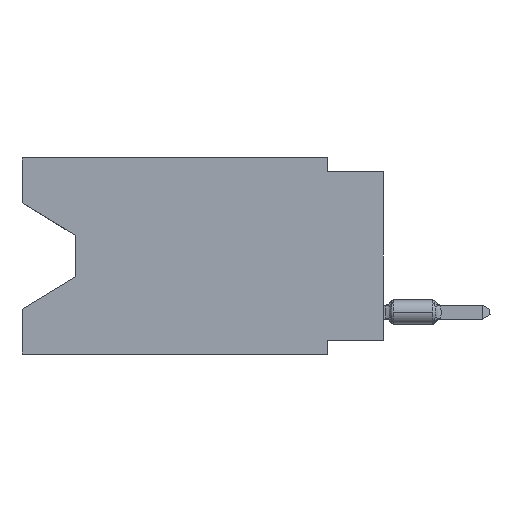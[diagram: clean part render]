
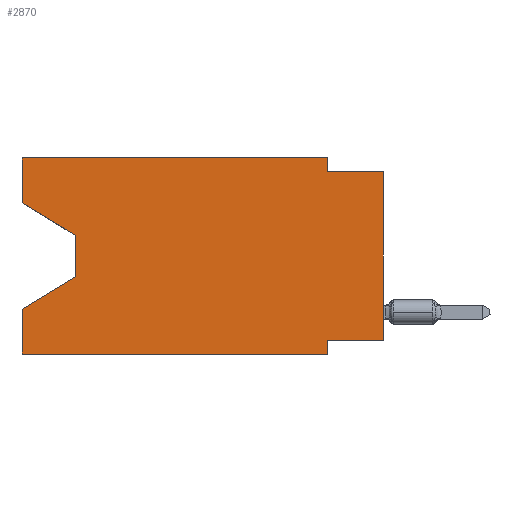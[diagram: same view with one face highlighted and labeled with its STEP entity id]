
A CAD part, left-side view. The second image highlights one B-rep face of the part: STEP entity #2870.
In plain terms, the highlighted planar face has unit normal (-1, 0, 0).
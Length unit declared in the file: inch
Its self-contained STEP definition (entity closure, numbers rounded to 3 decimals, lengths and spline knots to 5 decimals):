
#119 = CARTESIAN_POINT ( 'NONE',  ( 0., 0., -0.025 ) ) ;
#227 = DIRECTION ( 'NONE',  ( 0., 1., 0. ) ) ;
#538 = CARTESIAN_POINT ( 'NONE',  ( 0., 0.645, 0. ) ) ;
#648 = VERTEX_POINT ( 'NONE', #4481 ) ;
#923 = LINE ( 'NONE', #16245, #11190 ) ;
#1853 = VERTEX_POINT ( 'NONE', #9119 ) ;
#1995 = ORIENTED_EDGE ( 'NONE', *, *, #6807, .F. ) ;
#2394 = DIRECTION ( 'NONE',  ( 0., 0., 1. ) ) ;
#2590 = CARTESIAN_POINT ( 'NONE',  ( 0., 0.1, 0. ) ) ;
#2631 = VECTOR ( 'NONE', #4880, 39.37008 ) ;
#2761 = ORIENTED_EDGE ( 'NONE', *, *, #10690, .F. ) ;
#2870 = ADVANCED_FACE ( 'NONE', ( #11526 ), #4623, .F. ) ;
#3121 = LINE ( 'NONE', #119, #16254 ) ;
#3537 = CARTESIAN_POINT ( 'NONE',  ( 0., 0.55, -0.212 ) ) ;
#3776 = LINE ( 'NONE', #10771, #2631 ) ;
#4215 = EDGE_CURVE ( 'NONE', #14684, #5134, #6753, .T. ) ;
#4271 = CARTESIAN_POINT ( 'NONE',  ( 0., 0.645, 0. ) ) ;
#4279 = ORIENTED_EDGE ( 'NONE', *, *, #12678, .F. ) ;
#4481 = CARTESIAN_POINT ( 'NONE',  ( 0., 0.645, -0.08025 ) ) ;
#4498 = DIRECTION ( 'NONE',  ( 0., -1., 0. ) ) ;
#4530 = DIRECTION ( 'NONE',  ( 0., 0., -1. ) ) ;
#4623 = PLANE ( 'NONE',  #16631 ) ;
#4880 = DIRECTION ( 'NONE',  ( 0., 0., 1. ) ) ;
#4951 = CARTESIAN_POINT ( 'NONE',  ( 0., 0.1, -0.35 ) ) ;
#5134 = VERTEX_POINT ( 'NONE', #6136 ) ;
#5175 = CARTESIAN_POINT ( 'NONE',  ( 0., 0.645, -0.35 ) ) ;
#5552 = ORIENTED_EDGE ( 'NONE', *, *, #16722, .T. ) ;
#5636 = VECTOR ( 'NONE', #7919, 39.37008 ) ;
#5731 = EDGE_CURVE ( 'NONE', #13386, #7227, #6645, .T. ) ;
#6094 = CARTESIAN_POINT ( 'NONE',  ( 0., 0.55, -0.138 ) ) ;
#6136 = CARTESIAN_POINT ( 'NONE',  ( 0., 0.645, -0.26975 ) ) ;
#6188 = VERTEX_POINT ( 'NONE', #2590 ) ;
#6567 = CARTESIAN_POINT ( 'NONE',  ( 0., 0.645, 0. ) ) ;
#6645 = LINE ( 'NONE', #16562, #5636 ) ;
#6753 = LINE ( 'NONE', #3537, #9103 ) ;
#6807 = EDGE_CURVE ( 'NONE', #6920, #6188, #11647, .T. ) ;
#6920 = VERTEX_POINT ( 'NONE', #6567 ) ;
#7227 = VERTEX_POINT ( 'NONE', #4951 ) ;
#7360 = DIRECTION ( 'NONE',  ( 1., 0., 0. ) ) ;
#7716 = ORIENTED_EDGE ( 'NONE', *, *, #11211, .T. ) ;
#7802 = ORIENTED_EDGE ( 'NONE', *, *, #4215, .T. ) ;
#7919 = DIRECTION ( 'NONE',  ( 0., 0., -1. ) ) ;
#8076 = LINE ( 'NONE', #13598, #15418 ) ;
#8245 = CARTESIAN_POINT ( 'NONE',  ( 0., 0.1, -0.325 ) ) ;
#8449 = CARTESIAN_POINT ( 'NONE',  ( 0., 0.55, -0.138 ) ) ;
#9063 = ORIENTED_EDGE ( 'NONE', *, *, #5731, .F. ) ;
#9103 = VECTOR ( 'NONE', #17960, 39.37008 ) ;
#9119 = CARTESIAN_POINT ( 'NONE',  ( 0., 0., -0.325 ) ) ;
#9915 = ORIENTED_EDGE ( 'NONE', *, *, #12034, .F. ) ;
#10001 = EDGE_CURVE ( 'NONE', #1853, #14406, #8076, .T. ) ;
#10349 = VECTOR ( 'NONE', #17234, 39.37008 ) ;
#10369 = CARTESIAN_POINT ( 'NONE',  ( 0., 0., -0.025 ) ) ;
#10690 = EDGE_CURVE ( 'NONE', #12665, #14406, #3121, .T. ) ;
#10771 = CARTESIAN_POINT ( 'NONE',  ( 0., 0.645, 0. ) ) ;
#11175 = EDGE_CURVE ( 'NONE', #648, #6920, #16847, .T. ) ;
#11190 = VECTOR ( 'NONE', #16158, 39.37008 ) ;
#11211 = EDGE_CURVE ( 'NONE', #12664, #7227, #17116, .T. ) ;
#11329 = CARTESIAN_POINT ( 'NONE',  ( 0., 0., -0.325 ) ) ;
#11416 = LINE ( 'NONE', #11329, #14553 ) ;
#11526 = FACE_OUTER_BOUND ( 'NONE', #13293, .T. ) ;
#11647 = LINE ( 'NONE', #538, #10349 ) ;
#11814 = DIRECTION ( 'NONE',  ( 0., 0., -1. ) ) ;
#11896 = VECTOR ( 'NONE', #11814, 39.37008 ) ;
#11991 = CARTESIAN_POINT ( 'NONE',  ( 0., 0.1, 0. ) ) ;
#12034 = EDGE_CURVE ( 'NONE', #6188, #12665, #13463, .T. ) ;
#12065 = ORIENTED_EDGE ( 'NONE', *, *, #16146, .F. ) ;
#12164 = ORIENTED_EDGE ( 'NONE', *, *, #11175, .F. ) ;
#12369 = EDGE_CURVE ( 'NONE', #16475, #14684, #13174, .T. ) ;
#12617 = CARTESIAN_POINT ( 'NONE',  ( 0., 0.1, -0.025 ) ) ;
#12620 = CARTESIAN_POINT ( 'NONE',  ( 0., 0.55, -0.212 ) ) ;
#12664 = VERTEX_POINT ( 'NONE', #5175 ) ;
#12665 = VERTEX_POINT ( 'NONE', #12617 ) ;
#12678 = EDGE_CURVE ( 'NONE', #1853, #13386, #11416, .T. ) ;
#12985 = DIRECTION ( 'NONE',  ( 0., 0., 1. ) ) ;
#13174 = LINE ( 'NONE', #6094, #17470 ) ;
#13293 = EDGE_LOOP ( 'NONE', ( #5552, #14595, #7802, #12065, #7716, #9063, #4279, #16386, #2761, #9915, #1995, #12164 ) ) ;
#13386 = VERTEX_POINT ( 'NONE', #8245 ) ;
#13463 = LINE ( 'NONE', #11991, #11896 ) ;
#13598 = CARTESIAN_POINT ( 'NONE',  ( 0., 0., 0. ) ) ;
#14354 = CARTESIAN_POINT ( 'NONE',  ( 0., 0.645, -0.35 ) ) ;
#14406 = VERTEX_POINT ( 'NONE', #10369 ) ;
#14553 = VECTOR ( 'NONE', #227, 39.37008 ) ;
#14595 = ORIENTED_EDGE ( 'NONE', *, *, #12369, .T. ) ;
#14629 = CARTESIAN_POINT ( 'NONE',  ( 0., 0.645, 0. ) ) ;
#14684 = VERTEX_POINT ( 'NONE', #12620 ) ;
#14793 = VECTOR ( 'NONE', #17475, 39.37008 ) ;
#14809 = DIRECTION ( 'NONE',  ( 0., 0., -1. ) ) ;
#15418 = VECTOR ( 'NONE', #2394, 39.37008 ) ;
#16146 = EDGE_CURVE ( 'NONE', #12664, #5134, #3776, .T. ) ;
#16158 = DIRECTION ( 'NONE',  ( 0., -0.855, -0.519 ) ) ;
#16245 = CARTESIAN_POINT ( 'NONE',  ( 0., 0.645, -0.08025 ) ) ;
#16254 = VECTOR ( 'NONE', #4498, 39.37008 ) ;
#16386 = ORIENTED_EDGE ( 'NONE', *, *, #10001, .T. ) ;
#16475 = VERTEX_POINT ( 'NONE', #8449 ) ;
#16562 = CARTESIAN_POINT ( 'NONE',  ( 0., 0.1, -0.35 ) ) ;
#16631 = AXIS2_PLACEMENT_3D ( 'NONE', #14629, #7360, #4530 ) ;
#16722 = EDGE_CURVE ( 'NONE', #648, #16475, #923, .T. ) ;
#16847 = LINE ( 'NONE', #4271, #18035 ) ;
#17116 = LINE ( 'NONE', #14354, #14793 ) ;
#17234 = DIRECTION ( 'NONE',  ( 0., -1., 0. ) ) ;
#17470 = VECTOR ( 'NONE', #14809, 39.37008 ) ;
#17475 = DIRECTION ( 'NONE',  ( 0., -1., 0. ) ) ;
#17960 = DIRECTION ( 'NONE',  ( 0., 0.855, -0.519 ) ) ;
#18035 = VECTOR ( 'NONE', #12985, 39.37008 ) ;
